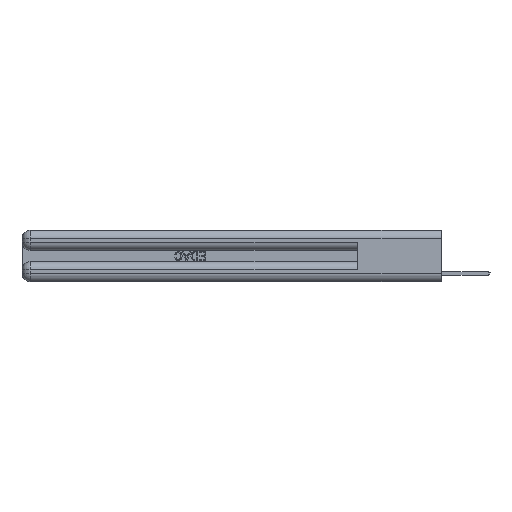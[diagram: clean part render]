
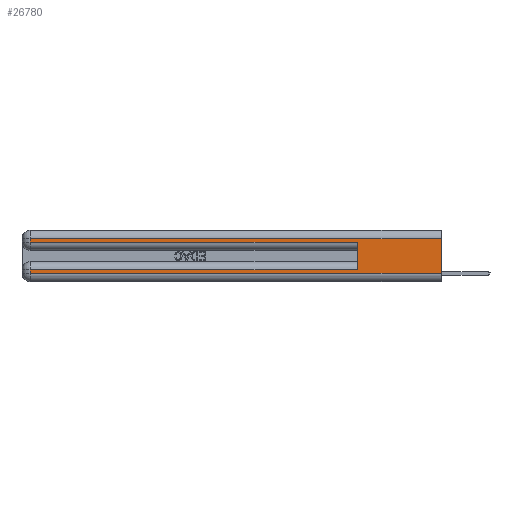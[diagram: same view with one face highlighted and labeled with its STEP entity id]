
A CAD part, left-side view. The second image highlights one B-rep face of the part: STEP entity #26780.
In plain terms, the highlighted planar face has unit normal (-1, 0, 0).
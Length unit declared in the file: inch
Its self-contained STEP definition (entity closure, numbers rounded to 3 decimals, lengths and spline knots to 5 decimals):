
#1 = LINE ( 'NONE', #3428, #29834 ) ;
#250 = VECTOR ( 'NONE', #8633, 39.37008 ) ;
#627 = ORIENTED_EDGE ( 'NONE', *, *, #29649, .T. ) ;
#900 = VERTEX_POINT ( 'NONE', #29831 ) ;
#1038 = LINE ( 'NONE', #2122, #12738 ) ;
#2122 = CARTESIAN_POINT ( 'NONE',  ( 0., 2.94, 0.37 ) ) ;
#2483 = LINE ( 'NONE', #27906, #23572 ) ;
#3160 = CARTESIAN_POINT ( 'NONE',  ( 0., 2.94, 0.285 ) ) ;
#3428 = CARTESIAN_POINT ( 'NONE',  ( 0., 0., 0.31 ) ) ;
#4708 = ORIENTED_EDGE ( 'NONE', *, *, #19815, .T. ) ;
#4966 = LINE ( 'NONE', #31107, #17019 ) ;
#5803 = CARTESIAN_POINT ( 'NONE',  ( 0., 2.94, 0.31 ) ) ;
#5996 = LINE ( 'NONE', #22955, #13957 ) ;
#6203 = ORIENTED_EDGE ( 'NONE', *, *, #6252, .T. ) ;
#6252 = EDGE_CURVE ( 'NONE', #6380, #26532, #1038, .T. ) ;
#6380 = VERTEX_POINT ( 'NONE', #5803 ) ;
#6704 = EDGE_CURVE ( 'NONE', #900, #18879, #2483, .T. ) ;
#8478 = CARTESIAN_POINT ( 'NONE',  ( 0., 0., 0.06 ) ) ;
#8559 = DIRECTION ( 'NONE',  ( 0., -1., 0. ) ) ;
#8633 = DIRECTION ( 'NONE',  ( 0., 0., 1. ) ) ;
#8683 = CARTESIAN_POINT ( 'NONE',  ( 0., 0., 0.37 ) ) ;
#8968 = PLANE ( 'NONE',  #18891 ) ;
#11747 = ORIENTED_EDGE ( 'NONE', *, *, #12427, .T. ) ;
#12234 = VERTEX_POINT ( 'NONE', #13009 ) ;
#12427 = EDGE_CURVE ( 'NONE', #18879, #24337, #5996, .T. ) ;
#12723 = CARTESIAN_POINT ( 'NONE',  ( 0., 2.94, 0.06 ) ) ;
#12738 = VECTOR ( 'NONE', #31255, 39.37008 ) ;
#13009 = CARTESIAN_POINT ( 'NONE',  ( 0., 0.6, 0.285 ) ) ;
#13073 = EDGE_CURVE ( 'NONE', #25385, #12234, #18760, .T. ) ;
#13132 = DIRECTION ( 'NONE',  ( 0., 0., -1. ) ) ;
#13843 = DIRECTION ( 'NONE',  ( 0., 0., -1. ) ) ;
#13957 = VECTOR ( 'NONE', #8559, 39.37008 ) ;
#14522 = VECTOR ( 'NONE', #27904, 39.37008 ) ;
#17019 = VECTOR ( 'NONE', #18763, 39.37008 ) ;
#17389 = VERTEX_POINT ( 'NONE', #23040 ) ;
#18312 = CARTESIAN_POINT ( 'NONE',  ( 0., 0.6, 0.145 ) ) ;
#18542 = EDGE_CURVE ( 'NONE', #25385, #900, #20908, .T. ) ;
#18652 = DIRECTION ( 'NONE',  ( 1., 0., 0. ) ) ;
#18760 = LINE ( 'NONE', #18312, #250 ) ;
#18763 = DIRECTION ( 'NONE',  ( 0., -1., 0. ) ) ;
#18879 = VERTEX_POINT ( 'NONE', #12723 ) ;
#18891 = AXIS2_PLACEMENT_3D ( 'NONE', #28256, #18652, #13843 ) ;
#19356 = CARTESIAN_POINT ( 'NONE',  ( 0., 0.6, 0.085 ) ) ;
#19645 = DIRECTION ( 'NONE',  ( 0., 0., -1. ) ) ;
#19815 = EDGE_CURVE ( 'NONE', #26532, #12234, #4966, .T. ) ;
#20081 = FACE_OUTER_BOUND ( 'NONE', #31115, .T. ) ;
#20908 = LINE ( 'NONE', #25156, #14522 ) ;
#21474 = ORIENTED_EDGE ( 'NONE', *, *, #13073, .F. ) ;
#22955 = CARTESIAN_POINT ( 'NONE',  ( 0., 0., 0.06 ) ) ;
#23040 = CARTESIAN_POINT ( 'NONE',  ( 0., 0., 0.31 ) ) ;
#23572 = VECTOR ( 'NONE', #19645, 39.37008 ) ;
#24109 = LINE ( 'NONE', #8683, #26919 ) ;
#24337 = VERTEX_POINT ( 'NONE', #8478 ) ;
#25156 = CARTESIAN_POINT ( 'NONE',  ( 0., 0., 0.085 ) ) ;
#25385 = VERTEX_POINT ( 'NONE', #19356 ) ;
#26532 = VERTEX_POINT ( 'NONE', #3160 ) ;
#26780 = ADVANCED_FACE ( 'NONE', ( #20081 ), #8968, .F. ) ;
#26919 = VECTOR ( 'NONE', #13132, 39.37008 ) ;
#27534 = ORIENTED_EDGE ( 'NONE', *, *, #28587, .F. ) ;
#27904 = DIRECTION ( 'NONE',  ( 0., 1., 0. ) ) ;
#27906 = CARTESIAN_POINT ( 'NONE',  ( 0., 2.94, 0.37 ) ) ;
#28256 = CARTESIAN_POINT ( 'NONE',  ( 0., 0., 0.37 ) ) ;
#28587 = EDGE_CURVE ( 'NONE', #17389, #24337, #24109, .T. ) ;
#28955 = ORIENTED_EDGE ( 'NONE', *, *, #18542, .T. ) ;
#29326 = ORIENTED_EDGE ( 'NONE', *, *, #6704, .T. ) ;
#29649 = EDGE_CURVE ( 'NONE', #17389, #6380, #1, .T. ) ;
#29831 = CARTESIAN_POINT ( 'NONE',  ( 0., 2.94, 0.085 ) ) ;
#29834 = VECTOR ( 'NONE', #29931, 39.37008 ) ;
#29931 = DIRECTION ( 'NONE',  ( 0., 1., 0. ) ) ;
#31107 = CARTESIAN_POINT ( 'NONE',  ( 0., 0., 0.285 ) ) ;
#31115 = EDGE_LOOP ( 'NONE', ( #27534, #627, #6203, #4708, #21474, #28955, #29326, #11747 ) ) ;
#31255 = DIRECTION ( 'NONE',  ( 0., 0., -1. ) ) ;
